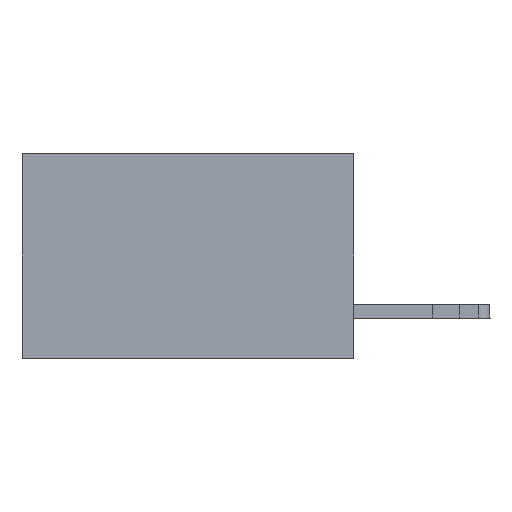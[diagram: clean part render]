
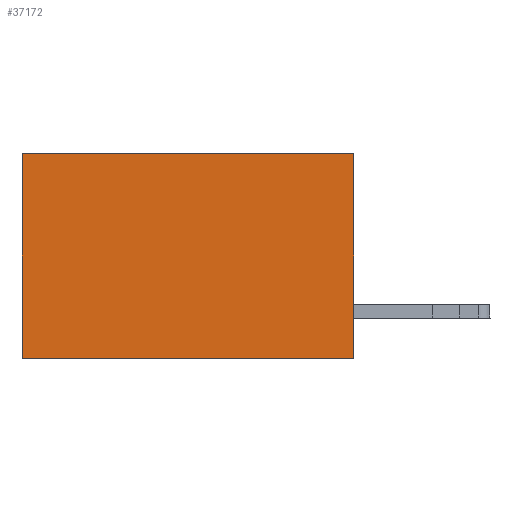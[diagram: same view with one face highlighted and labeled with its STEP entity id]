
A CAD part, left-side view. The second image highlights one B-rep face of the part: STEP entity #37172.
In plain terms, the highlighted planar face has unit normal (-1, 0, 0).
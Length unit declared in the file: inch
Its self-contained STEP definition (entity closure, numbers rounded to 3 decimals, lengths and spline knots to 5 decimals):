
#219 = VECTOR ( 'NONE', #4395, 39.37008 ) ;
#417 = FACE_OUTER_BOUND ( 'NONE', #38650, .T. ) ;
#1840 = VECTOR ( 'NONE', #38434, 39.37008 ) ;
#2079 = LINE ( 'NONE', #10987, #34809 ) ;
#4395 = DIRECTION ( 'NONE',  ( 0., 1., 0. ) ) ;
#7364 = LINE ( 'NONE', #31289, #219 ) ;
#8008 = EDGE_CURVE ( 'NONE', #10337, #12844, #19930, .T. ) ;
#8898 = EDGE_CURVE ( 'NONE', #10337, #37421, #2079, .T. ) ;
#9510 = CARTESIAN_POINT ( 'NONE',  ( 0.2875, 0., 0. ) ) ;
#10337 = VERTEX_POINT ( 'NONE', #35630 ) ;
#10987 = CARTESIAN_POINT ( 'NONE',  ( 0.2875, 0., 0. ) ) ;
#11646 = ORIENTED_EDGE ( 'NONE', *, *, #8898, .T. ) ;
#12503 = PLANE ( 'NONE',  #33379 ) ;
#12844 = VERTEX_POINT ( 'NONE', #31902 ) ;
#14385 = DIRECTION ( 'NONE',  ( 0., 1., 0. ) ) ;
#16750 = CARTESIAN_POINT ( 'NONE',  ( 0.2875, 0., 0. ) ) ;
#19013 = CARTESIAN_POINT ( 'NONE',  ( 0.2875, 0.6, 0. ) ) ;
#19930 = LINE ( 'NONE', #16750, #1840 ) ;
#21419 = VERTEX_POINT ( 'NONE', #29240 ) ;
#22112 = EDGE_CURVE ( 'NONE', #37421, #21419, #29969, .T. ) ;
#24530 = ORIENTED_EDGE ( 'NONE', *, *, #22112, .T. ) ;
#24664 = DIRECTION ( 'NONE',  ( 1., 0., 0. ) ) ;
#24958 = DIRECTION ( 'NONE',  ( 0., 0., -1. ) ) ;
#28804 = VECTOR ( 'NONE', #24958, 39.37008 ) ;
#29240 = CARTESIAN_POINT ( 'NONE',  ( 0.2875, 0.6, -0.37 ) ) ;
#29969 = LINE ( 'NONE', #19013, #28804 ) ;
#31289 = CARTESIAN_POINT ( 'NONE',  ( 0.2875, 0., -0.37 ) ) ;
#31706 = ORIENTED_EDGE ( 'NONE', *, *, #33299, .F. ) ;
#31902 = CARTESIAN_POINT ( 'NONE',  ( 0.2875, 0., -0.37 ) ) ;
#33299 = EDGE_CURVE ( 'NONE', #12844, #21419, #7364, .T. ) ;
#33379 = AXIS2_PLACEMENT_3D ( 'NONE', #9510, #24664, #33818 ) ;
#33818 = DIRECTION ( 'NONE',  ( 0., 0., -1. ) ) ;
#34809 = VECTOR ( 'NONE', #14385, 39.37008 ) ;
#35630 = CARTESIAN_POINT ( 'NONE',  ( 0.2875, 0., 0. ) ) ;
#36163 = ORIENTED_EDGE ( 'NONE', *, *, #8008, .F. ) ;
#37172 = ADVANCED_FACE ( 'NONE', ( #417 ), #12503, .F. ) ;
#37421 = VERTEX_POINT ( 'NONE', #37773 ) ;
#37773 = CARTESIAN_POINT ( 'NONE',  ( 0.2875, 0.6, 0. ) ) ;
#38434 = DIRECTION ( 'NONE',  ( 0., 0., -1. ) ) ;
#38650 = EDGE_LOOP ( 'NONE', ( #24530, #31706, #36163, #11646 ) ) ;
